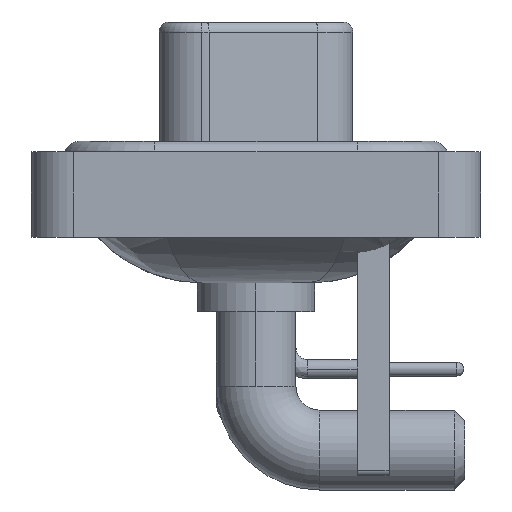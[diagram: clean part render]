
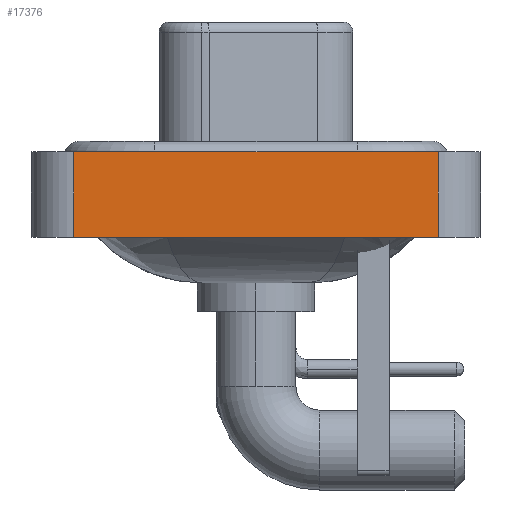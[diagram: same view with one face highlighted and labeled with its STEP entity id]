
A CAD part, left-side view. The second image highlights one B-rep face of the part: STEP entity #17376.
In plain terms, the highlighted planar face has unit normal (-1, 0, 0).
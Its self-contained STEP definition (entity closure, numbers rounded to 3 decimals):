
#516 = LINE ( 'NONE', #25140, #11410 ) ;
#1253 = FACE_OUTER_BOUND ( 'NONE', #7882, .T. ) ;
#2766 = CARTESIAN_POINT ( 'NONE',  ( -7.35, 8.55, 0.4 ) ) ;
#4420 = CARTESIAN_POINT ( 'NONE',  ( -7.35, -8.55, 0.4 ) ) ;
#5246 = VECTOR ( 'NONE', #5980, 1000. ) ;
#5255 = DIRECTION ( 'NONE',  ( -1., 0., 0. ) ) ;
#5455 = CARTESIAN_POINT ( 'NONE',  ( -7.35, 8.55, -3.6 ) ) ;
#5980 = DIRECTION ( 'NONE',  ( 0., 0., 1. ) ) ;
#6098 = DIRECTION ( 'NONE',  ( 0., -1., 0. ) ) ;
#7419 = VECTOR ( 'NONE', #6098, 1000. ) ;
#7882 = EDGE_LOOP ( 'NONE', ( #17944, #17303, #29173, #11936 ) ) ;
#9325 = EDGE_CURVE ( 'NONE', #15438, #14404, #19420, .T. ) ;
#9544 = EDGE_CURVE ( 'NONE', #16313, #26299, #516, .T. ) ;
#9651 = VECTOR ( 'NONE', #12559, 1000. ) ;
#11410 = VECTOR ( 'NONE', #11888, 1000. ) ;
#11888 = DIRECTION ( 'NONE',  ( 0., 0., 1. ) ) ;
#11936 = ORIENTED_EDGE ( 'NONE', *, *, #24814, .T. ) ;
#12489 = CARTESIAN_POINT ( 'NONE',  ( -7.35, -8.55, -3.6 ) ) ;
#12559 = DIRECTION ( 'NONE',  ( 0., -1., 0. ) ) ;
#14391 = CARTESIAN_POINT ( 'NONE',  ( -7.35, -8.55, -3.6 ) ) ;
#14404 = VERTEX_POINT ( 'NONE', #2766 ) ;
#15382 = CARTESIAN_POINT ( 'NONE',  ( -7.35, -8.55, 0.4 ) ) ;
#15438 = VERTEX_POINT ( 'NONE', #5455 ) ;
#16313 = VERTEX_POINT ( 'NONE', #12489 ) ;
#17188 = CARTESIAN_POINT ( 'NONE',  ( -7.35, 8.55, -3.6 ) ) ;
#17303 = ORIENTED_EDGE ( 'NONE', *, *, #28641, .F. ) ;
#17376 = ADVANCED_FACE ( 'NONE', ( #1253 ), #21157, .T. ) ;
#17734 = LINE ( 'NONE', #15382, #7419 ) ;
#17944 = ORIENTED_EDGE ( 'NONE', *, *, #9544, .T. ) ;
#19420 = LINE ( 'NONE', #17188, #5246 ) ;
#19467 = LINE ( 'NONE', #23440, #9651 ) ;
#21157 = PLANE ( 'NONE',  #24701 ) ;
#23440 = CARTESIAN_POINT ( 'NONE',  ( -7.35, -8.55, -3.6 ) ) ;
#24701 = AXIS2_PLACEMENT_3D ( 'NONE', #14391, #5255, #25593 ) ;
#24814 = EDGE_CURVE ( 'NONE', #15438, #16313, #19467, .T. ) ;
#25140 = CARTESIAN_POINT ( 'NONE',  ( -7.35, -8.55, -3.6 ) ) ;
#25593 = DIRECTION ( 'NONE',  ( 0., 0., 1. ) ) ;
#26299 = VERTEX_POINT ( 'NONE', #4420 ) ;
#28641 = EDGE_CURVE ( 'NONE', #14404, #26299, #17734, .T. ) ;
#29173 = ORIENTED_EDGE ( 'NONE', *, *, #9325, .F. ) ;
